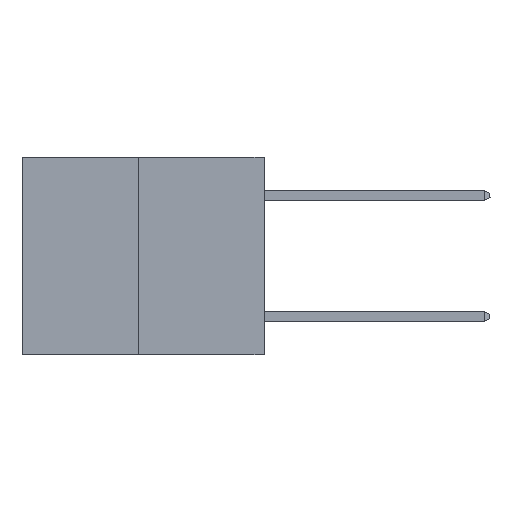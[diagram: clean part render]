
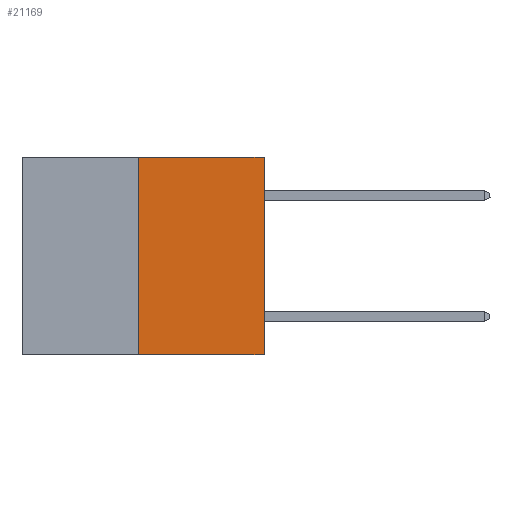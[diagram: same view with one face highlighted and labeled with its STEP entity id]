
A CAD part, left-side view. The second image highlights one B-rep face of the part: STEP entity #21169.
In plain terms, the highlighted planar face has unit normal (-1, 0, 0).
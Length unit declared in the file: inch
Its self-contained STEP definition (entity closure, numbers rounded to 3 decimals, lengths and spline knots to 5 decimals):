
#36 = CARTESIAN_POINT ( 'NONE',  ( 0., 0.6, 0. ) ) ;
#590 = PLANE ( 'NONE',  #29763 ) ;
#2766 = VECTOR ( 'NONE', #30786, 39.37008 ) ;
#4265 = CARTESIAN_POINT ( 'NONE',  ( 0., 0., 0. ) ) ;
#4580 = VERTEX_POINT ( 'NONE', #23228 ) ;
#5806 = CARTESIAN_POINT ( 'NONE',  ( 0., 0.312, -0.49 ) ) ;
#6965 = EDGE_CURVE ( 'NONE', #26751, #21132, #7022, .T. ) ;
#7022 = LINE ( 'NONE', #36, #28227 ) ;
#7984 = DIRECTION ( 'NONE',  ( 1., 0., 0. ) ) ;
#8043 = CARTESIAN_POINT ( 'NONE',  ( 0., 0.312, 0. ) ) ;
#8732 = EDGE_LOOP ( 'NONE', ( #22883, #16050, #27119, #26018 ) ) ;
#8750 = DIRECTION ( 'NONE',  ( 0., -1., 0. ) ) ;
#9013 = VECTOR ( 'NONE', #8750, 39.37008 ) ;
#9042 = CARTESIAN_POINT ( 'NONE',  ( 0., 0.6, -0.49 ) ) ;
#9960 = CARTESIAN_POINT ( 'NONE',  ( 0., 0., 0. ) ) ;
#10558 = CARTESIAN_POINT ( 'NONE',  ( 0., 0.312, -0.49 ) ) ;
#11961 = EDGE_CURVE ( 'NONE', #29884, #4580, #22624, .T. ) ;
#13900 = LINE ( 'NONE', #5806, #19556 ) ;
#15582 = LINE ( 'NONE', #4265, #2766 ) ;
#16050 = ORIENTED_EDGE ( 'NONE', *, *, #11961, .T. ) ;
#19556 = VECTOR ( 'NONE', #30030, 39.37008 ) ;
#21132 = VERTEX_POINT ( 'NONE', #9960 ) ;
#21169 = ADVANCED_FACE ( 'NONE', ( #25645 ), #590, .F. ) ;
#21654 = DIRECTION ( 'NONE',  ( 0., -1., 0. ) ) ;
#22624 = LINE ( 'NONE', #9042, #9013 ) ;
#22883 = ORIENTED_EDGE ( 'NONE', *, *, #27994, .F. ) ;
#23228 = CARTESIAN_POINT ( 'NONE',  ( 0., 0., -0.49 ) ) ;
#25645 = FACE_OUTER_BOUND ( 'NONE', #8732, .T. ) ;
#25817 = EDGE_CURVE ( 'NONE', #4580, #21132, #15582, .T. ) ;
#26018 = ORIENTED_EDGE ( 'NONE', *, *, #6965, .F. ) ;
#26751 = VERTEX_POINT ( 'NONE', #8043 ) ;
#27119 = ORIENTED_EDGE ( 'NONE', *, *, #25817, .T. ) ;
#27994 = EDGE_CURVE ( 'NONE', #29884, #26751, #13900, .T. ) ;
#28227 = VECTOR ( 'NONE', #21654, 39.37008 ) ;
#29763 = AXIS2_PLACEMENT_3D ( 'NONE', #30132, #7984, #29820 ) ;
#29820 = DIRECTION ( 'NONE',  ( 0., 0., -1. ) ) ;
#29884 = VERTEX_POINT ( 'NONE', #10558 ) ;
#30030 = DIRECTION ( 'NONE',  ( 0., 0., 1. ) ) ;
#30132 = CARTESIAN_POINT ( 'NONE',  ( 0., 0.6, 0. ) ) ;
#30786 = DIRECTION ( 'NONE',  ( 0., 0., 1. ) ) ;
